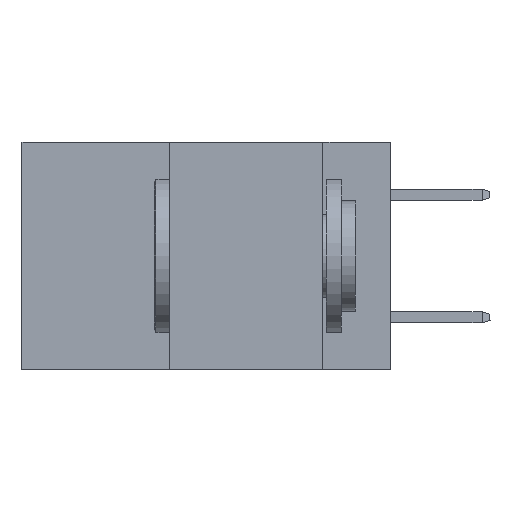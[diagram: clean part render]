
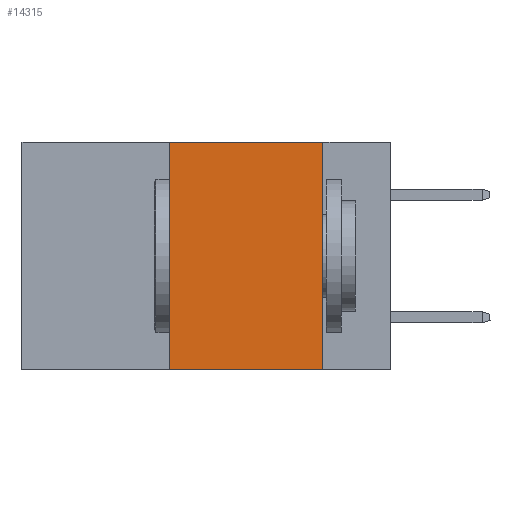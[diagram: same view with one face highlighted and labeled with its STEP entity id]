
A CAD part, left-side view. The second image highlights one B-rep face of the part: STEP entity #14315.
In plain terms, the highlighted planar face has unit normal (-1, 0, 0).
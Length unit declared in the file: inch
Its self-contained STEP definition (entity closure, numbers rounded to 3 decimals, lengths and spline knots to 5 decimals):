
#242 = DIRECTION ( 'NONE',  ( 0., -1., 0. ) ) ;
#626 = CARTESIAN_POINT ( 'NONE',  ( 0., 0.11, 0. ) ) ;
#702 = DIRECTION ( 'NONE',  ( 1., 0., 0. ) ) ;
#803 = VECTOR ( 'NONE', #8297, 39.37008 ) ;
#981 = ORIENTED_EDGE ( 'NONE', *, *, #6184, .F. ) ;
#1191 = VERTEX_POINT ( 'NONE', #626 ) ;
#1950 = CARTESIAN_POINT ( 'NONE',  ( 0., 0.6, 0. ) ) ;
#3133 = EDGE_CURVE ( 'NONE', #5949, #11549, #5451, .T. ) ;
#4644 = LINE ( 'NONE', #1950, #13448 ) ;
#5307 = FACE_OUTER_BOUND ( 'NONE', #18054, .T. ) ;
#5451 = LINE ( 'NONE', #11754, #803 ) ;
#5507 = VECTOR ( 'NONE', #10479, 39.37008 ) ;
#5949 = VERTEX_POINT ( 'NONE', #15690 ) ;
#6039 = VECTOR ( 'NONE', #17914, 39.37008 ) ;
#6051 = DIRECTION ( 'NONE',  ( 0., 0., -1. ) ) ;
#6184 = EDGE_CURVE ( 'NONE', #1191, #14734, #16831, .T. ) ;
#6468 = ORIENTED_EDGE ( 'NONE', *, *, #8331, .T. ) ;
#8297 = DIRECTION ( 'NONE',  ( 0., 0., 1. ) ) ;
#8331 = EDGE_CURVE ( 'NONE', #5949, #14734, #12361, .T. ) ;
#10479 = DIRECTION ( 'NONE',  ( 0., 0., -1. ) ) ;
#10623 = ORIENTED_EDGE ( 'NONE', *, *, #18722, .F. ) ;
#10721 = AXIS2_PLACEMENT_3D ( 'NONE', #16636, #702, #6051 ) ;
#11549 = VERTEX_POINT ( 'NONE', #14402 ) ;
#11754 = CARTESIAN_POINT ( 'NONE',  ( 0., 0.36, 0. ) ) ;
#12361 = LINE ( 'NONE', #17847, #6039 ) ;
#13448 = VECTOR ( 'NONE', #242, 39.37008 ) ;
#14315 = ADVANCED_FACE ( 'NONE', ( #5307 ), #15009, .F. ) ;
#14402 = CARTESIAN_POINT ( 'NONE',  ( 0., 0.36, 0. ) ) ;
#14734 = VERTEX_POINT ( 'NONE', #20891 ) ;
#15009 = PLANE ( 'NONE',  #10721 ) ;
#15690 = CARTESIAN_POINT ( 'NONE',  ( 0., 0.36, -0.37 ) ) ;
#16636 = CARTESIAN_POINT ( 'NONE',  ( 0., 0.6, 0. ) ) ;
#16831 = LINE ( 'NONE', #19254, #5507 ) ;
#16891 = ORIENTED_EDGE ( 'NONE', *, *, #3133, .F. ) ;
#17847 = CARTESIAN_POINT ( 'NONE',  ( 0., 0.6, -0.37 ) ) ;
#17914 = DIRECTION ( 'NONE',  ( 0., -1., 0. ) ) ;
#18054 = EDGE_LOOP ( 'NONE', ( #981, #10623, #16891, #6468 ) ) ;
#18722 = EDGE_CURVE ( 'NONE', #11549, #1191, #4644, .T. ) ;
#19254 = CARTESIAN_POINT ( 'NONE',  ( 0., 0.11, 0. ) ) ;
#20891 = CARTESIAN_POINT ( 'NONE',  ( 0., 0.11, -0.37 ) ) ;
